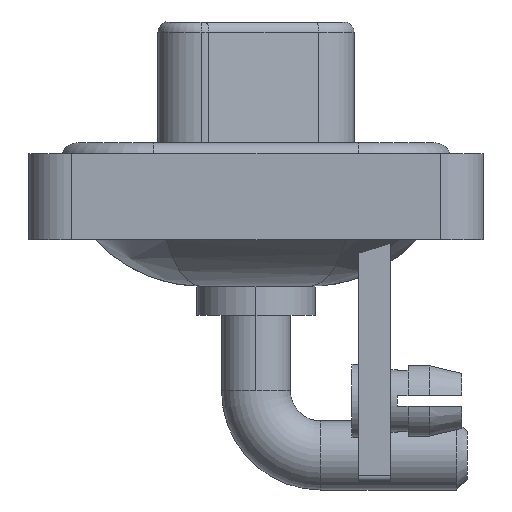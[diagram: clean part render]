
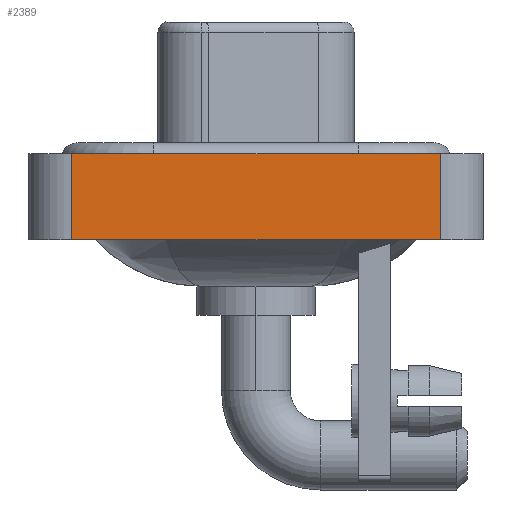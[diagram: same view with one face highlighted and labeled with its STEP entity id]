
A CAD part, left-side view. The second image highlights one B-rep face of the part: STEP entity #2389.
In plain terms, the highlighted planar face has unit normal (-1, 0, 0).
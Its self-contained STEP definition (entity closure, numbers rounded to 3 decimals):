
#9 = EDGE_CURVE ( 'NONE', #13257, #7530, #2878, .T. ) ;
#177 = AXIS2_PLACEMENT_3D ( 'NONE', #7535, #13095, #10336 ) ;
#574 = EDGE_CURVE ( 'NONE', #17906, #7530, #937, .T. ) ;
#937 = LINE ( 'NONE', #3606, #7403 ) ;
#2389 = ADVANCED_FACE ( 'NONE', ( #3185 ), #17663, .T. ) ;
#2805 = ORIENTED_EDGE ( 'NONE', *, *, #9, .T. ) ;
#2878 = LINE ( 'NONE', #9047, #8274 ) ;
#3185 = FACE_OUTER_BOUND ( 'NONE', #10974, .T. ) ;
#3606 = CARTESIAN_POINT ( 'NONE',  ( -7.3, -8.55, 0.4 ) ) ;
#4581 = DIRECTION ( 'NONE',  ( 0., 0., 1. ) ) ;
#5066 = CARTESIAN_POINT ( 'NONE',  ( -7.3, 8.55, -3.6 ) ) ;
#5524 = VECTOR ( 'NONE', #14843, 1000. ) ;
#6312 = EDGE_CURVE ( 'NONE', #17923, #17906, #18036, .T. ) ;
#7287 = CARTESIAN_POINT ( 'NONE',  ( -7.3, -8.55, -3.6 ) ) ;
#7403 = VECTOR ( 'NONE', #14095, 1000. ) ;
#7530 = VERTEX_POINT ( 'NONE', #13314 ) ;
#7535 = CARTESIAN_POINT ( 'NONE',  ( -7.3, -8.55, -3.6 ) ) ;
#8274 = VECTOR ( 'NONE', #4581, 1000. ) ;
#8315 = ORIENTED_EDGE ( 'NONE', *, *, #6312, .F. ) ;
#9047 = CARTESIAN_POINT ( 'NONE',  ( -7.3, -8.55, -3.6 ) ) ;
#9416 = EDGE_CURVE ( 'NONE', #17923, #13257, #16274, .T. ) ;
#10336 = DIRECTION ( 'NONE',  ( 0., 0., 1. ) ) ;
#10895 = DIRECTION ( 'NONE',  ( 0., 0., 1. ) ) ;
#10974 = EDGE_LOOP ( 'NONE', ( #2805, #15419, #8315, #11776 ) ) ;
#11467 = CARTESIAN_POINT ( 'NONE',  ( -7.3, -8.55, -3.6 ) ) ;
#11585 = VECTOR ( 'NONE', #10895, 1000. ) ;
#11776 = ORIENTED_EDGE ( 'NONE', *, *, #9416, .T. ) ;
#13095 = DIRECTION ( 'NONE',  ( -1., 0., 0. ) ) ;
#13257 = VERTEX_POINT ( 'NONE', #11467 ) ;
#13314 = CARTESIAN_POINT ( 'NONE',  ( -7.3, -8.55, 0.4 ) ) ;
#14095 = DIRECTION ( 'NONE',  ( 0., -1., 0. ) ) ;
#14843 = DIRECTION ( 'NONE',  ( 0., -1., 0. ) ) ;
#15419 = ORIENTED_EDGE ( 'NONE', *, *, #574, .F. ) ;
#16274 = LINE ( 'NONE', #7287, #5524 ) ;
#16927 = CARTESIAN_POINT ( 'NONE',  ( -7.3, 8.55, 0.4 ) ) ;
#17663 = PLANE ( 'NONE',  #177 ) ;
#17906 = VERTEX_POINT ( 'NONE', #16927 ) ;
#17923 = VERTEX_POINT ( 'NONE', #18267 ) ;
#18036 = LINE ( 'NONE', #5066, #11585 ) ;
#18267 = CARTESIAN_POINT ( 'NONE',  ( -7.3, 8.55, -3.6 ) ) ;
